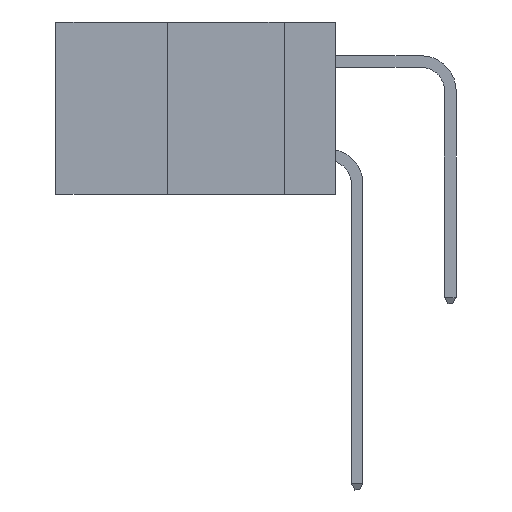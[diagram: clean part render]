
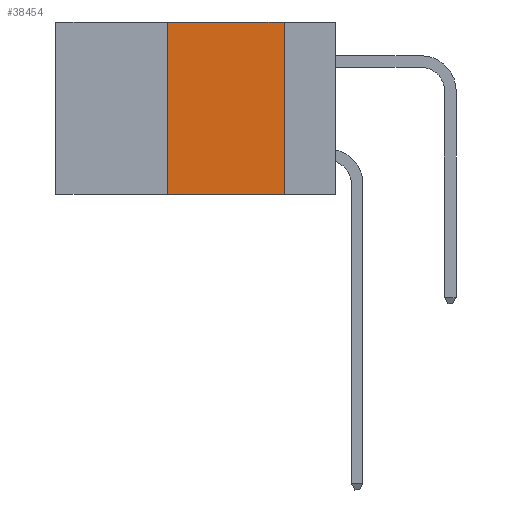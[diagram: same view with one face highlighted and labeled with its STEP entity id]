
A CAD part, left-side view. The second image highlights one B-rep face of the part: STEP entity #38454.
In plain terms, the highlighted planar face has unit normal (-1, 0, 0).
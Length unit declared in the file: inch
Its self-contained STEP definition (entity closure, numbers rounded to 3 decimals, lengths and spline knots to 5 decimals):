
#698 = LINE ( 'NONE', #26756, #7930 ) ;
#2548 = CARTESIAN_POINT ( 'NONE',  ( 0., 0.6, 0. ) ) ;
#2853 = ORIENTED_EDGE ( 'NONE', *, *, #30825, .F. ) ;
#3019 = CARTESIAN_POINT ( 'NONE',  ( 0., 0.11, -0.37 ) ) ;
#3235 = ORIENTED_EDGE ( 'NONE', *, *, #35825, .T. ) ;
#4690 = DIRECTION ( 'NONE',  ( 0., -1., 0. ) ) ;
#6405 = DIRECTION ( 'NONE',  ( 0., 0., -1. ) ) ;
#6623 = CARTESIAN_POINT ( 'NONE',  ( 0., 0.36, 0. ) ) ;
#7930 = VECTOR ( 'NONE', #6405, 39.37008 ) ;
#8580 = VERTEX_POINT ( 'NONE', #38542 ) ;
#9680 = DIRECTION ( 'NONE',  ( 0., 0., 1. ) ) ;
#13273 = VERTEX_POINT ( 'NONE', #19965 ) ;
#13480 = LINE ( 'NONE', #2548, #24810 ) ;
#13889 = CARTESIAN_POINT ( 'NONE',  ( 0., 0.6, -0.37 ) ) ;
#14711 = ORIENTED_EDGE ( 'NONE', *, *, #16834, .F. ) ;
#15528 = ORIENTED_EDGE ( 'NONE', *, *, #19027, .F. ) ;
#16834 = EDGE_CURVE ( 'NONE', #27850, #17169, #698, .T. ) ;
#17169 = VERTEX_POINT ( 'NONE', #3019 ) ;
#19027 = EDGE_CURVE ( 'NONE', #13273, #27850, #13480, .T. ) ;
#19887 = AXIS2_PLACEMENT_3D ( 'NONE', #38609, #30037, #20488 ) ;
#19965 = CARTESIAN_POINT ( 'NONE',  ( 0., 0.36, 0. ) ) ;
#20484 = VECTOR ( 'NONE', #9680, 39.37008 ) ;
#20488 = DIRECTION ( 'NONE',  ( 0., 0., -1. ) ) ;
#21790 = LINE ( 'NONE', #13889, #35103 ) ;
#22059 = FACE_OUTER_BOUND ( 'NONE', #26118, .T. ) ;
#24810 = VECTOR ( 'NONE', #32884, 39.37008 ) ;
#26118 = EDGE_LOOP ( 'NONE', ( #14711, #15528, #2853, #3235 ) ) ;
#26756 = CARTESIAN_POINT ( 'NONE',  ( 0., 0.11, 0. ) ) ;
#26959 = PLANE ( 'NONE',  #19887 ) ;
#27850 = VERTEX_POINT ( 'NONE', #27990 ) ;
#27990 = CARTESIAN_POINT ( 'NONE',  ( 0., 0.11, 0. ) ) ;
#28561 = LINE ( 'NONE', #6623, #20484 ) ;
#30037 = DIRECTION ( 'NONE',  ( 1., 0., 0. ) ) ;
#30825 = EDGE_CURVE ( 'NONE', #8580, #13273, #28561, .T. ) ;
#32884 = DIRECTION ( 'NONE',  ( 0., -1., 0. ) ) ;
#35103 = VECTOR ( 'NONE', #4690, 39.37008 ) ;
#35825 = EDGE_CURVE ( 'NONE', #8580, #17169, #21790, .T. ) ;
#38454 = ADVANCED_FACE ( 'NONE', ( #22059 ), #26959, .F. ) ;
#38542 = CARTESIAN_POINT ( 'NONE',  ( 0., 0.36, -0.37 ) ) ;
#38609 = CARTESIAN_POINT ( 'NONE',  ( 0., 0.6, 0. ) ) ;
